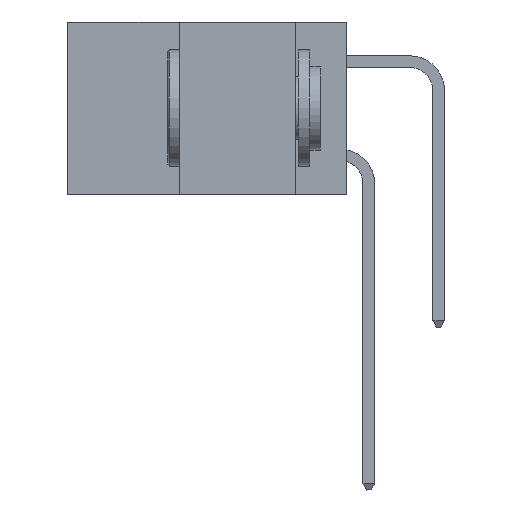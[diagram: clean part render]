
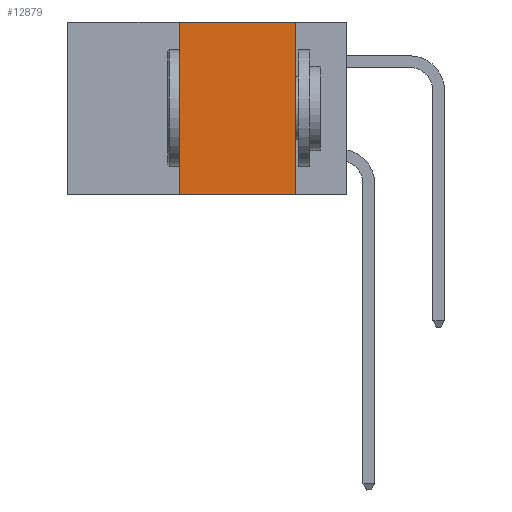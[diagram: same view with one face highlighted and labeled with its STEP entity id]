
A CAD part, left-side view. The second image highlights one B-rep face of the part: STEP entity #12879.
In plain terms, the highlighted planar face has unit normal (-1, 0, 0).
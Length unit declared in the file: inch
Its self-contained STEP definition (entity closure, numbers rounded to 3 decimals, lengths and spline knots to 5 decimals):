
#115 = DIRECTION ( 'NONE',  ( 0., 0., -1. ) ) ;
#512 = EDGE_CURVE ( 'NONE', #5486, #9522, #9227, .T. ) ;
#1870 = PLANE ( 'NONE',  #8539 ) ;
#3149 = DIRECTION ( 'NONE',  ( 0., 0., 1. ) ) ;
#3526 = VERTEX_POINT ( 'NONE', #11818 ) ;
#3588 = DIRECTION ( 'NONE',  ( 0., 0., -1. ) ) ;
#4016 = CARTESIAN_POINT ( 'NONE',  ( 0., 0.6, 0. ) ) ;
#4216 = CARTESIAN_POINT ( 'NONE',  ( 0., 0.11, -0.37 ) ) ;
#4981 = ORIENTED_EDGE ( 'NONE', *, *, #17804, .F. ) ;
#5144 = DIRECTION ( 'NONE',  ( 0., -1., 0. ) ) ;
#5270 = VECTOR ( 'NONE', #5144, 39.37008 ) ;
#5486 = VERTEX_POINT ( 'NONE', #18623 ) ;
#7478 = DIRECTION ( 'NONE',  ( 0., -1., 0. ) ) ;
#8539 = AXIS2_PLACEMENT_3D ( 'NONE', #16686, #13565, #3588 ) ;
#8730 = LINE ( 'NONE', #4016, #12004 ) ;
#8831 = EDGE_LOOP ( 'NONE', ( #16992, #17487, #4981, #13765 ) ) ;
#9227 = LINE ( 'NONE', #20735, #5270 ) ;
#9233 = FACE_OUTER_BOUND ( 'NONE', #8831, .T. ) ;
#9522 = VERTEX_POINT ( 'NONE', #4216 ) ;
#9901 = CARTESIAN_POINT ( 'NONE',  ( 0., 0.36, 0. ) ) ;
#11068 = CARTESIAN_POINT ( 'NONE',  ( 0., 0.11, 0. ) ) ;
#11818 = CARTESIAN_POINT ( 'NONE',  ( 0., 0.36, 0. ) ) ;
#11893 = CARTESIAN_POINT ( 'NONE',  ( 0., 0.11, 0. ) ) ;
#12004 = VECTOR ( 'NONE', #7478, 39.37008 ) ;
#12046 = VECTOR ( 'NONE', #115, 39.37008 ) ;
#12099 = LINE ( 'NONE', #9901, #19948 ) ;
#12879 = ADVANCED_FACE ( 'NONE', ( #9233 ), #1870, .F. ) ;
#13565 = DIRECTION ( 'NONE',  ( 1., 0., 0. ) ) ;
#13765 = ORIENTED_EDGE ( 'NONE', *, *, #512, .T. ) ;
#16686 = CARTESIAN_POINT ( 'NONE',  ( 0., 0.6, 0. ) ) ;
#16992 = ORIENTED_EDGE ( 'NONE', *, *, #19065, .F. ) ;
#17487 = ORIENTED_EDGE ( 'NONE', *, *, #20418, .F. ) ;
#17804 = EDGE_CURVE ( 'NONE', #5486, #3526, #12099, .T. ) ;
#18623 = CARTESIAN_POINT ( 'NONE',  ( 0., 0.36, -0.37 ) ) ;
#18751 = VERTEX_POINT ( 'NONE', #11068 ) ;
#19065 = EDGE_CURVE ( 'NONE', #18751, #9522, #20374, .T. ) ;
#19948 = VECTOR ( 'NONE', #3149, 39.37008 ) ;
#20374 = LINE ( 'NONE', #11893, #12046 ) ;
#20418 = EDGE_CURVE ( 'NONE', #3526, #18751, #8730, .T. ) ;
#20735 = CARTESIAN_POINT ( 'NONE',  ( 0., 0.6, -0.37 ) ) ;
